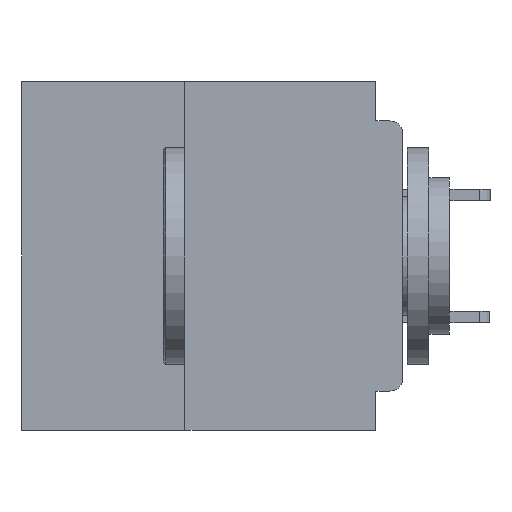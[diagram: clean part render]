
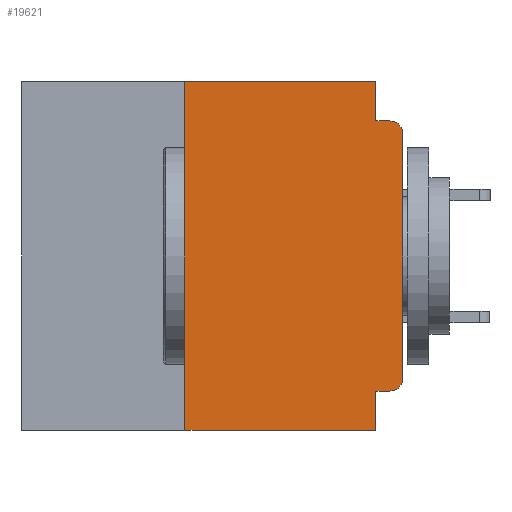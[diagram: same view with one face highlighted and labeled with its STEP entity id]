
A CAD part, left-side view. The second image highlights one B-rep face of the part: STEP entity #19621.
In plain terms, the highlighted planar face has unit normal (-1, 0, 0).
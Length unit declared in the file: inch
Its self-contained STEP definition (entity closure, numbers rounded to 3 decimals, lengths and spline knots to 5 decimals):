
#486 = VECTOR ( 'NONE', #44617, 39.37008 ) ;
#3296 = VERTEX_POINT ( 'NONE', #17776 ) ;
#5144 = ORIENTED_EDGE ( 'NONE', *, *, #17737, .F. ) ;
#5369 = PLANE ( 'NONE',  #25175 ) ;
#7343 = LINE ( 'NONE', #31390, #17446 ) ;
#8009 = ORIENTED_EDGE ( 'NONE', *, *, #17378, .F. ) ;
#8344 = ORIENTED_EDGE ( 'NONE', *, *, #16139, .F. ) ;
#8669 = LINE ( 'NONE', #46630, #18729 ) ;
#8862 = ORIENTED_EDGE ( 'NONE', *, *, #18171, .F. ) ;
#9951 = DIRECTION ( 'NONE',  ( 0., 0., -1. ) ) ;
#11797 = CIRCLE ( 'NONE', #18870, 0.015 ) ;
#12450 = EDGE_CURVE ( 'NONE', #14102, #17680, #45468, .T. ) ;
#12766 = CARTESIAN_POINT ( 'NONE',  ( 0., 0.25, 0. ) ) ;
#13845 = CARTESIAN_POINT ( 'NONE',  ( 0., 0., -0.355 ) ) ;
#14102 = VERTEX_POINT ( 'NONE', #26549 ) ;
#14406 = CARTESIAN_POINT ( 'NONE',  ( 0., 0.015, -0.045 ) ) ;
#14525 = AXIS2_PLACEMENT_3D ( 'NONE', #19269, #48785, #23514 ) ;
#15156 = VERTEX_POINT ( 'NONE', #54168 ) ;
#15329 = ORIENTED_EDGE ( 'NONE', *, *, #48902, .F. ) ;
#15514 = VECTOR ( 'NONE', #25837, 39.37008 ) ;
#16139 = EDGE_CURVE ( 'NONE', #3296, #28788, #42087, .T. ) ;
#16374 = CARTESIAN_POINT ( 'NONE',  ( 0., 0.031, -0.4 ) ) ;
#17031 = ORIENTED_EDGE ( 'NONE', *, *, #20306, .T. ) ;
#17070 = LINE ( 'NONE', #45870, #36940 ) ;
#17130 = EDGE_CURVE ( 'NONE', #47479, #15156, #26784, .T. ) ;
#17319 = CARTESIAN_POINT ( 'NONE',  ( 0., 0., 0. ) ) ;
#17378 = EDGE_CURVE ( 'NONE', #22190, #46727, #34717, .T. ) ;
#17446 = VECTOR ( 'NONE', #39829, 39.37008 ) ;
#17680 = VERTEX_POINT ( 'NONE', #26834 ) ;
#17737 = EDGE_CURVE ( 'NONE', #54979, #22190, #7343, .T. ) ;
#17776 = CARTESIAN_POINT ( 'NONE',  ( 0., 0.015, -0.355 ) ) ;
#18125 = CIRCLE ( 'NONE', #14525, 0.015 ) ;
#18171 = EDGE_CURVE ( 'NONE', #46727, #18386, #8669, .T. ) ;
#18386 = VERTEX_POINT ( 'NONE', #14406 ) ;
#18505 = ORIENTED_EDGE ( 'NONE', *, *, #17130, .T. ) ;
#18729 = VECTOR ( 'NONE', #42561, 39.37008 ) ;
#18870 = AXIS2_PLACEMENT_3D ( 'NONE', #45315, #20032, #49527 ) ;
#19269 = CARTESIAN_POINT ( 'NONE',  ( 0., 0.015, -0.06 ) ) ;
#19621 = ADVANCED_FACE ( 'NONE', ( #41346 ), #5369, .F. ) ;
#20032 = DIRECTION ( 'NONE',  ( -1., 0., 0. ) ) ;
#20306 = EDGE_CURVE ( 'NONE', #15156, #18386, #18125, .T. ) ;
#22190 = VERTEX_POINT ( 'NONE', #53475 ) ;
#23195 = CARTESIAN_POINT ( 'NONE',  ( 0., 0.437, -0.4 ) ) ;
#23452 = EDGE_CURVE ( 'NONE', #3296, #47479, #11797, .T. ) ;
#23514 = DIRECTION ( 'NONE',  ( 0., 0., -1. ) ) ;
#24832 = DIRECTION ( 'NONE',  ( 0., 0., 1. ) ) ;
#25175 = AXIS2_PLACEMENT_3D ( 'NONE', #47932, #35433, #9951 ) ;
#25348 = LINE ( 'NONE', #16374, #47783 ) ;
#25837 = DIRECTION ( 'NONE',  ( 0., 0., 1. ) ) ;
#26549 = CARTESIAN_POINT ( 'NONE',  ( 0., 0.25, -0.4 ) ) ;
#26784 = LINE ( 'NONE', #17319, #15514 ) ;
#26834 = CARTESIAN_POINT ( 'NONE',  ( 0., 0.031, -0.4 ) ) ;
#27358 = CARTESIAN_POINT ( 'NONE',  ( 0., 0., -0.34 ) ) ;
#28261 = ORIENTED_EDGE ( 'NONE', *, *, #23452, .T. ) ;
#28788 = VERTEX_POINT ( 'NONE', #38581 ) ;
#31390 = CARTESIAN_POINT ( 'NONE',  ( 0., 0.437, 0. ) ) ;
#32230 = VECTOR ( 'NONE', #43459, 39.37008 ) ;
#34280 = VECTOR ( 'NONE', #48468, 39.37008 ) ;
#34717 = LINE ( 'NONE', #40375, #486 ) ;
#34740 = EDGE_CURVE ( 'NONE', #28788, #17680, #25348, .T. ) ;
#35433 = DIRECTION ( 'NONE',  ( 1., 0., 0. ) ) ;
#36940 = VECTOR ( 'NONE', #24832, 39.37008 ) ;
#37098 = ORIENTED_EDGE ( 'NONE', *, *, #12450, .T. ) ;
#38581 = CARTESIAN_POINT ( 'NONE',  ( 0., 0.031, -0.355 ) ) ;
#39829 = DIRECTION ( 'NONE',  ( 0., -1., 0. ) ) ;
#40375 = CARTESIAN_POINT ( 'NONE',  ( 0., 0.031, 0. ) ) ;
#41346 = FACE_OUTER_BOUND ( 'NONE', #49290, .T. ) ;
#42087 = LINE ( 'NONE', #13845, #32230 ) ;
#42561 = DIRECTION ( 'NONE',  ( 0., -1., 0. ) ) ;
#43459 = DIRECTION ( 'NONE',  ( 0., 1., 0. ) ) ;
#43708 = ORIENTED_EDGE ( 'NONE', *, *, #34740, .F. ) ;
#44617 = DIRECTION ( 'NONE',  ( 0., 0., -1. ) ) ;
#45315 = CARTESIAN_POINT ( 'NONE',  ( 0., 0.015, -0.34 ) ) ;
#45468 = LINE ( 'NONE', #23195, #34280 ) ;
#45870 = CARTESIAN_POINT ( 'NONE',  ( 0., 0.25, -0.4 ) ) ;
#45921 = DIRECTION ( 'NONE',  ( 0., 0., -1. ) ) ;
#46630 = CARTESIAN_POINT ( 'NONE',  ( 0., 0., -0.045 ) ) ;
#46727 = VERTEX_POINT ( 'NONE', #51581 ) ;
#47479 = VERTEX_POINT ( 'NONE', #27358 ) ;
#47783 = VECTOR ( 'NONE', #45921, 39.37008 ) ;
#47932 = CARTESIAN_POINT ( 'NONE',  ( 0., 0.437, 0. ) ) ;
#48468 = DIRECTION ( 'NONE',  ( 0., -1., 0. ) ) ;
#48785 = DIRECTION ( 'NONE',  ( -1., 0., 0. ) ) ;
#48902 = EDGE_CURVE ( 'NONE', #14102, #54979, #17070, .T. ) ;
#49290 = EDGE_LOOP ( 'NONE', ( #18505, #17031, #8862, #8009, #5144, #15329, #37098, #43708, #8344, #28261 ) ) ;
#49527 = DIRECTION ( 'NONE',  ( 0., 0., -1. ) ) ;
#51581 = CARTESIAN_POINT ( 'NONE',  ( 0., 0.031, -0.045 ) ) ;
#53475 = CARTESIAN_POINT ( 'NONE',  ( 0., 0.031, 0. ) ) ;
#54168 = CARTESIAN_POINT ( 'NONE',  ( 0., 0., -0.06 ) ) ;
#54979 = VERTEX_POINT ( 'NONE', #12766 ) ;
